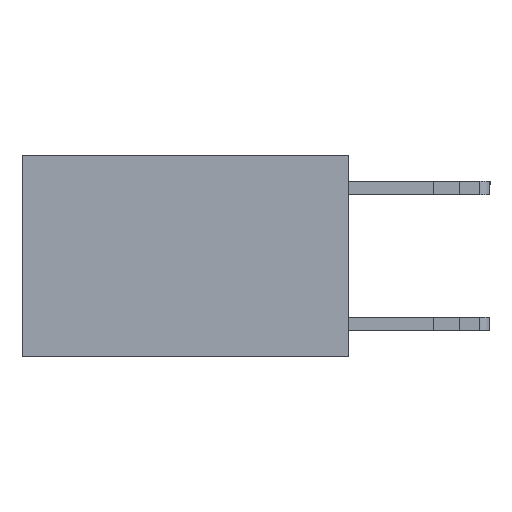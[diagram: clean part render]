
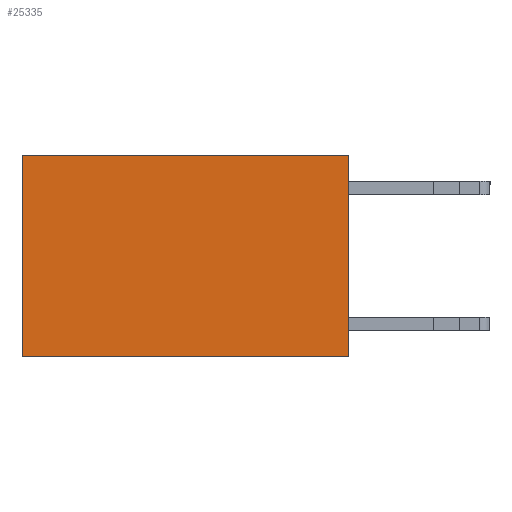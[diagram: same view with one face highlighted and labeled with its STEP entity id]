
A CAD part, left-side view. The second image highlights one B-rep face of the part: STEP entity #25335.
In plain terms, the highlighted planar face has unit normal (-1, 0, 0).
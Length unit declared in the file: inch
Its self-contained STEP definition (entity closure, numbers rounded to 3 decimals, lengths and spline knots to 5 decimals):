
#980 = VECTOR ( 'NONE', #8636, 39.37008 ) ;
#1160 = CARTESIAN_POINT ( 'NONE',  ( 0.2625, 0., -0.37 ) ) ;
#2092 = CARTESIAN_POINT ( 'NONE',  ( 0.2625, 0., -0.37 ) ) ;
#2411 = VECTOR ( 'NONE', #15360, 39.37008 ) ;
#2471 = PLANE ( 'NONE',  #12159 ) ;
#3731 = LINE ( 'NONE', #6096, #8542 ) ;
#4005 = LINE ( 'NONE', #2092, #2411 ) ;
#5756 = VERTEX_POINT ( 'NONE', #9178 ) ;
#6096 = CARTESIAN_POINT ( 'NONE',  ( 0.2625, 0.6, 0. ) ) ;
#6150 = EDGE_CURVE ( 'NONE', #27904, #27810, #17127, .T. ) ;
#8108 = CARTESIAN_POINT ( 'NONE',  ( 0.2625, 0., 0. ) ) ;
#8492 = CARTESIAN_POINT ( 'NONE',  ( 0.2625, 0., 0. ) ) ;
#8542 = VECTOR ( 'NONE', #24406, 39.37008 ) ;
#8636 = DIRECTION ( 'NONE',  ( 0., 1., 0. ) ) ;
#8647 = EDGE_CURVE ( 'NONE', #15084, #5756, #3731, .T. ) ;
#8814 = DIRECTION ( 'NONE',  ( 1., 0., 0. ) ) ;
#9178 = CARTESIAN_POINT ( 'NONE',  ( 0.2625, 0.6, -0.37 ) ) ;
#10344 = EDGE_CURVE ( 'NONE', #27904, #15084, #15558, .T. ) ;
#10868 = FACE_OUTER_BOUND ( 'NONE', #23940, .T. ) ;
#12159 = AXIS2_PLACEMENT_3D ( 'NONE', #24624, #8814, #19873 ) ;
#12907 = ORIENTED_EDGE ( 'NONE', *, *, #6150, .F. ) ;
#14925 = CARTESIAN_POINT ( 'NONE',  ( 0.2625, 0., 0. ) ) ;
#15084 = VERTEX_POINT ( 'NONE', #21420 ) ;
#15360 = DIRECTION ( 'NONE',  ( 0., 1., 0. ) ) ;
#15558 = LINE ( 'NONE', #8492, #980 ) ;
#17127 = LINE ( 'NONE', #14925, #27529 ) ;
#19873 = DIRECTION ( 'NONE',  ( 0., 0., -1. ) ) ;
#21420 = CARTESIAN_POINT ( 'NONE',  ( 0.2625, 0.6, 0. ) ) ;
#22680 = ORIENTED_EDGE ( 'NONE', *, *, #28660, .F. ) ;
#23688 = ORIENTED_EDGE ( 'NONE', *, *, #8647, .T. ) ;
#23940 = EDGE_LOOP ( 'NONE', ( #23688, #22680, #12907, #24558 ) ) ;
#24406 = DIRECTION ( 'NONE',  ( 0., 0., -1. ) ) ;
#24558 = ORIENTED_EDGE ( 'NONE', *, *, #10344, .T. ) ;
#24624 = CARTESIAN_POINT ( 'NONE',  ( 0.2625, 0., 0. ) ) ;
#25335 = ADVANCED_FACE ( 'NONE', ( #10868 ), #2471, .F. ) ;
#27529 = VECTOR ( 'NONE', #29100, 39.37008 ) ;
#27810 = VERTEX_POINT ( 'NONE', #1160 ) ;
#27904 = VERTEX_POINT ( 'NONE', #8108 ) ;
#28660 = EDGE_CURVE ( 'NONE', #27810, #5756, #4005, .T. ) ;
#29100 = DIRECTION ( 'NONE',  ( 0., 0., -1. ) ) ;
